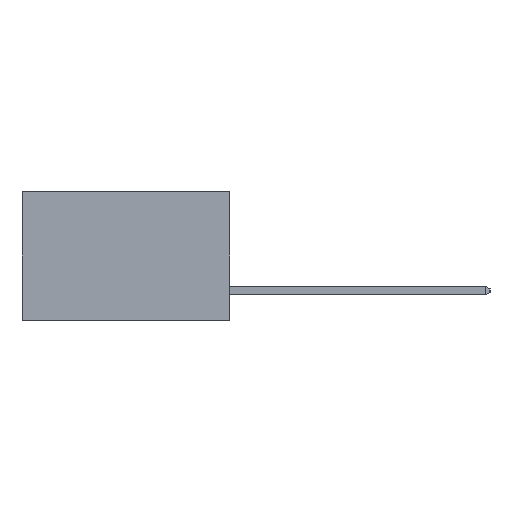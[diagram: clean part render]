
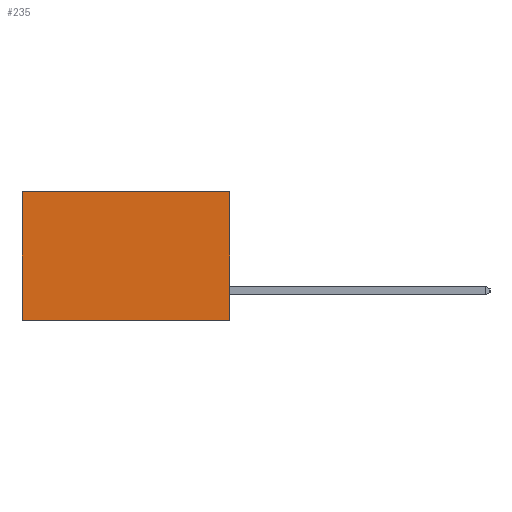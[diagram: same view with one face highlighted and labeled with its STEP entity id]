
A CAD part, left-side view. The second image highlights one B-rep face of the part: STEP entity #235.
In plain terms, the highlighted planar face has unit normal (-1, 0, 0).
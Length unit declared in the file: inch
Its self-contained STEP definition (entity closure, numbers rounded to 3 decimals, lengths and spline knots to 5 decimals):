
#34 = ORIENTED_EDGE ( 'NONE', *, *, #8636, .F. ) ;
#235 = ADVANCED_FACE ( 'NONE', ( #7216 ), #3597, .F. ) ;
#467 = ORIENTED_EDGE ( 'NONE', *, *, #10519, .T. ) ;
#634 = CARTESIAN_POINT ( 'NONE',  ( 0.298, 0.6, 0. ) ) ;
#696 = VERTEX_POINT ( 'NONE', #8608 ) ;
#1110 = DIRECTION ( 'NONE',  ( 0., 0., -1. ) ) ;
#1245 = CARTESIAN_POINT ( 'NONE',  ( 0.298, 0.6, 0. ) ) ;
#1747 = CARTESIAN_POINT ( 'NONE',  ( 0.298, 0., 0. ) ) ;
#1957 = VERTEX_POINT ( 'NONE', #1747 ) ;
#3071 = CARTESIAN_POINT ( 'NONE',  ( 0.298, 0.6, -0.37 ) ) ;
#3474 = EDGE_CURVE ( 'NONE', #1957, #696, #9906, .T. ) ;
#3479 = CARTESIAN_POINT ( 'NONE',  ( 0.298, 0., 0. ) ) ;
#3538 = VECTOR ( 'NONE', #1110, 39.37008 ) ;
#3560 = DIRECTION ( 'NONE',  ( 1., 0., 0. ) ) ;
#3597 = PLANE ( 'NONE',  #7622 ) ;
#3634 = DIRECTION ( 'NONE',  ( 0., 0., -1. ) ) ;
#4244 = LINE ( 'NONE', #6635, #5880 ) ;
#4572 = ORIENTED_EDGE ( 'NONE', *, *, #5043, .T. ) ;
#4813 = VERTEX_POINT ( 'NONE', #634 ) ;
#5043 = EDGE_CURVE ( 'NONE', #4813, #8039, #5707, .T. ) ;
#5524 = ORIENTED_EDGE ( 'NONE', *, *, #3474, .F. ) ;
#5540 = CARTESIAN_POINT ( 'NONE',  ( 0.298, 0., 0. ) ) ;
#5707 = LINE ( 'NONE', #1245, #3538 ) ;
#5880 = VECTOR ( 'NONE', #9806, 39.37008 ) ;
#6240 = VECTOR ( 'NONE', #9818, 39.37008 ) ;
#6635 = CARTESIAN_POINT ( 'NONE',  ( 0.298, 0., 0. ) ) ;
#7000 = DIRECTION ( 'NONE',  ( 0., 0., -1. ) ) ;
#7216 = FACE_OUTER_BOUND ( 'NONE', #7334, .T. ) ;
#7334 = EDGE_LOOP ( 'NONE', ( #4572, #34, #5524, #467 ) ) ;
#7622 = AXIS2_PLACEMENT_3D ( 'NONE', #3479, #3560, #3634 ) ;
#7776 = VECTOR ( 'NONE', #7000, 39.37008 ) ;
#8039 = VERTEX_POINT ( 'NONE', #3071 ) ;
#8608 = CARTESIAN_POINT ( 'NONE',  ( 0.298, 0., -0.37 ) ) ;
#8621 = LINE ( 'NONE', #9598, #6240 ) ;
#8636 = EDGE_CURVE ( 'NONE', #696, #8039, #8621, .T. ) ;
#9598 = CARTESIAN_POINT ( 'NONE',  ( 0.298, 0., -0.37 ) ) ;
#9806 = DIRECTION ( 'NONE',  ( 0., 1., 0. ) ) ;
#9818 = DIRECTION ( 'NONE',  ( 0., 1., 0. ) ) ;
#9906 = LINE ( 'NONE', #5540, #7776 ) ;
#10519 = EDGE_CURVE ( 'NONE', #1957, #4813, #4244, .T. ) ;
